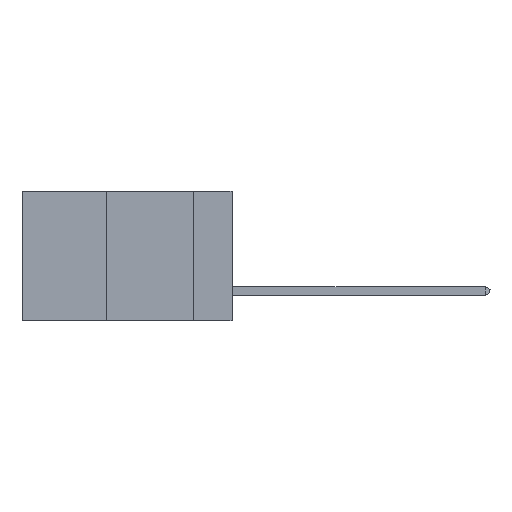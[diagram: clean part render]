
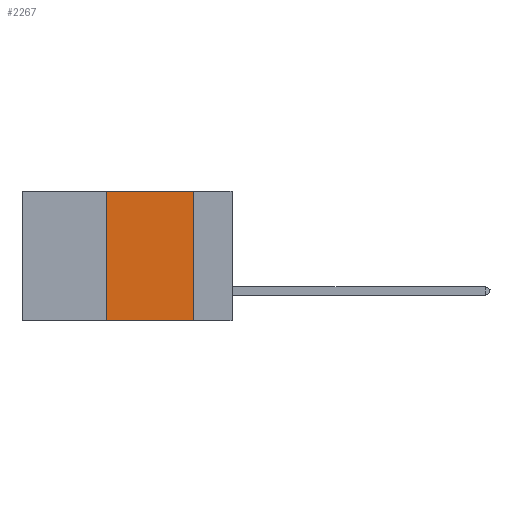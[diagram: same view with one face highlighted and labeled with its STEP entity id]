
A CAD part, left-side view. The second image highlights one B-rep face of the part: STEP entity #2267.
In plain terms, the highlighted planar face has unit normal (-1, 0, 0).
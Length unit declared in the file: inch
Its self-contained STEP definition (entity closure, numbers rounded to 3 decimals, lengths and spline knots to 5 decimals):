
#522 = ORIENTED_EDGE ( 'NONE', *, *, #9000, .T. ) ;
#1527 = CARTESIAN_POINT ( 'NONE',  ( 0., 0.36, 0. ) ) ;
#2267 = ADVANCED_FACE ( 'NONE', ( #2851 ), #10564, .F. ) ;
#2851 = FACE_OUTER_BOUND ( 'NONE', #16798, .T. ) ;
#3938 = EDGE_CURVE ( 'NONE', #19323, #8543, #23381, .T. ) ;
#4813 = CARTESIAN_POINT ( 'NONE',  ( 0., 0.11, 0. ) ) ;
#8543 = VERTEX_POINT ( 'NONE', #32462 ) ;
#9000 = EDGE_CURVE ( 'NONE', #32036, #8543, #23438, .T. ) ;
#9083 = ORIENTED_EDGE ( 'NONE', *, *, #3938, .F. ) ;
#9141 = VECTOR ( 'NONE', #13419, 39.37008 ) ;
#10564 = PLANE ( 'NONE',  #11008 ) ;
#10845 = ORIENTED_EDGE ( 'NONE', *, *, #18166, .F. ) ;
#10860 = EDGE_CURVE ( 'NONE', #21952, #19323, #23065, .T. ) ;
#11008 = AXIS2_PLACEMENT_3D ( 'NONE', #32202, #26992, #31846 ) ;
#11272 = LINE ( 'NONE', #26995, #9141 ) ;
#13419 = DIRECTION ( 'NONE',  ( 0., 0., 1. ) ) ;
#14723 = CARTESIAN_POINT ( 'NONE',  ( 0., 0.6, -0.37 ) ) ;
#15834 = VECTOR ( 'NONE', #21685, 39.37008 ) ;
#16223 = VECTOR ( 'NONE', #33703, 39.37008 ) ;
#16798 = EDGE_LOOP ( 'NONE', ( #9083, #25532, #10845, #522 ) ) ;
#18166 = EDGE_CURVE ( 'NONE', #32036, #21952, #11272, .T. ) ;
#19323 = VERTEX_POINT ( 'NONE', #4813 ) ;
#21685 = DIRECTION ( 'NONE',  ( 0., -1., 0. ) ) ;
#21952 = VERTEX_POINT ( 'NONE', #1527 ) ;
#22676 = CARTESIAN_POINT ( 'NONE',  ( 0., 0.11, 0. ) ) ;
#23065 = LINE ( 'NONE', #29411, #15834 ) ;
#23381 = LINE ( 'NONE', #22676, #30557 ) ;
#23438 = LINE ( 'NONE', #14723, #16223 ) ;
#25319 = DIRECTION ( 'NONE',  ( 0., 0., -1. ) ) ;
#25532 = ORIENTED_EDGE ( 'NONE', *, *, #10860, .F. ) ;
#26992 = DIRECTION ( 'NONE',  ( 1., 0., 0. ) ) ;
#26995 = CARTESIAN_POINT ( 'NONE',  ( 0., 0.36, 0. ) ) ;
#27636 = CARTESIAN_POINT ( 'NONE',  ( 0., 0.36, -0.37 ) ) ;
#29411 = CARTESIAN_POINT ( 'NONE',  ( 0., 0.6, 0. ) ) ;
#30557 = VECTOR ( 'NONE', #25319, 39.37008 ) ;
#31846 = DIRECTION ( 'NONE',  ( 0., 0., -1. ) ) ;
#32036 = VERTEX_POINT ( 'NONE', #27636 ) ;
#32202 = CARTESIAN_POINT ( 'NONE',  ( 0., 0.6, 0. ) ) ;
#32462 = CARTESIAN_POINT ( 'NONE',  ( 0., 0.11, -0.37 ) ) ;
#33703 = DIRECTION ( 'NONE',  ( 0., -1., 0. ) ) ;
